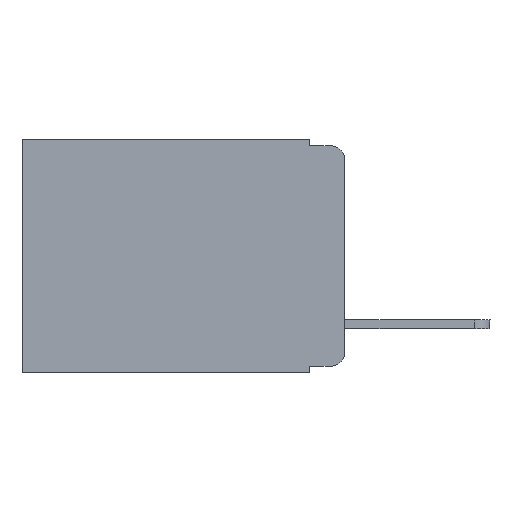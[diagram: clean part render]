
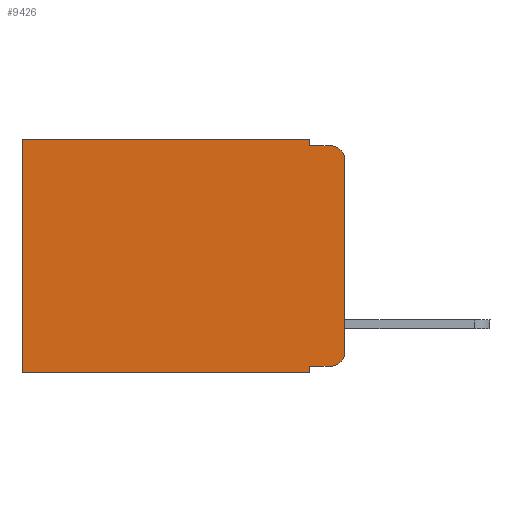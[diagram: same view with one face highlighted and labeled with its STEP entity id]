
A CAD part, left-side view. The second image highlights one B-rep face of the part: STEP entity #9426.
In plain terms, the highlighted planar face has unit normal (-1, 0, 0).
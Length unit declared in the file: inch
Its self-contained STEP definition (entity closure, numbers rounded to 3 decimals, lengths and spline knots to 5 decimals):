
#676 = LINE ( 'NONE', #734, #9993 ) ;
#734 = CARTESIAN_POINT ( 'NONE',  ( 0.298, 0.051, 0. ) ) ;
#769 = LINE ( 'NONE', #6448, #11673 ) ;
#831 = VERTEX_POINT ( 'NONE', #12209 ) ;
#836 = VERTEX_POINT ( 'NONE', #8332 ) ;
#1305 = AXIS2_PLACEMENT_3D ( 'NONE', #5976, #6216, #8032 ) ;
#1352 = CARTESIAN_POINT ( 'NONE',  ( 0.298, 0.473, -0.343 ) ) ;
#1422 = CARTESIAN_POINT ( 'NONE',  ( 0.298, 0.02, -0.01 ) ) ;
#1475 = VERTEX_POINT ( 'NONE', #4830 ) ;
#1585 = EDGE_CURVE ( 'NONE', #836, #831, #676, .T. ) ;
#1597 = DIRECTION ( 'NONE',  ( -1., 0., 0. ) ) ;
#1700 = EDGE_CURVE ( 'NONE', #8218, #3048, #10352, .T. ) ;
#1705 = VERTEX_POINT ( 'NONE', #7664 ) ;
#1864 = CARTESIAN_POINT ( 'NONE',  ( 0.298, 0., -0.313 ) ) ;
#1930 = DIRECTION ( 'NONE',  ( 0., 0., -1. ) ) ;
#2500 = DIRECTION ( 'NONE',  ( 0., 0., -1. ) ) ;
#2582 = DIRECTION ( 'NONE',  ( 0., 0., -1. ) ) ;
#2620 = AXIS2_PLACEMENT_3D ( 'NONE', #11358, #2967, #1930 ) ;
#2673 = CARTESIAN_POINT ( 'NONE',  ( 0.298, 0.051, -0.333 ) ) ;
#2722 = ORIENTED_EDGE ( 'NONE', *, *, #8827, .F. ) ;
#2781 = VECTOR ( 'NONE', #6067, 39.37008 ) ;
#2967 = DIRECTION ( 'NONE',  ( 1., 0., 0. ) ) ;
#3048 = VERTEX_POINT ( 'NONE', #1864 ) ;
#3181 = LINE ( 'NONE', #7083, #3971 ) ;
#3281 = VECTOR ( 'NONE', #6327, 39.37008 ) ;
#3443 = VERTEX_POINT ( 'NONE', #1422 ) ;
#3461 = VERTEX_POINT ( 'NONE', #10984 ) ;
#3486 = CARTESIAN_POINT ( 'NONE',  ( 0.298, 0.051, -0.01 ) ) ;
#3590 = PLANE ( 'NONE',  #2620 ) ;
#3823 = EDGE_CURVE ( 'NONE', #1705, #3443, #9048, .T. ) ;
#3971 = VECTOR ( 'NONE', #8991, 39.37008 ) ;
#4249 = CIRCLE ( 'NONE', #1305, 0.02 ) ;
#4801 = EDGE_CURVE ( 'NONE', #8218, #3443, #4249, .T. ) ;
#4830 = CARTESIAN_POINT ( 'NONE',  ( 0.298, 0.02, -0.333 ) ) ;
#5017 = LINE ( 'NONE', #11632, #2781 ) ;
#5194 = VECTOR ( 'NONE', #12122, 39.37008 ) ;
#5557 = LINE ( 'NONE', #11180, #10906 ) ;
#5901 = ORIENTED_EDGE ( 'NONE', *, *, #8743, .F. ) ;
#5976 = CARTESIAN_POINT ( 'NONE',  ( 0.298, 0.02, -0.03 ) ) ;
#6017 = CARTESIAN_POINT ( 'NONE',  ( 0.298, 0.051, 0. ) ) ;
#6067 = DIRECTION ( 'NONE',  ( 0., 1., 0. ) ) ;
#6143 = CIRCLE ( 'NONE', #8146, 0.02 ) ;
#6216 = DIRECTION ( 'NONE',  ( -1., 0., 0. ) ) ;
#6327 = DIRECTION ( 'NONE',  ( 0., -1., 0. ) ) ;
#6448 = CARTESIAN_POINT ( 'NONE',  ( 0.298, 0.051, 0. ) ) ;
#6751 = ORIENTED_EDGE ( 'NONE', *, *, #7006, .T. ) ;
#7006 = EDGE_CURVE ( 'NONE', #10038, #3461, #5017, .T. ) ;
#7079 = CARTESIAN_POINT ( 'NONE',  ( 0.298, 0., -0.03 ) ) ;
#7083 = CARTESIAN_POINT ( 'NONE',  ( 0.298, 0., -0.343 ) ) ;
#7356 = ORIENTED_EDGE ( 'NONE', *, *, #4801, .T. ) ;
#7437 = DIRECTION ( 'NONE',  ( 0., 0., -1. ) ) ;
#7639 = ORIENTED_EDGE ( 'NONE', *, *, #10543, .T. ) ;
#7664 = CARTESIAN_POINT ( 'NONE',  ( 0.298, 0.051, -0.01 ) ) ;
#7813 = VECTOR ( 'NONE', #9424, 39.37008 ) ;
#8032 = DIRECTION ( 'NONE',  ( 0., 0., -1. ) ) ;
#8146 = AXIS2_PLACEMENT_3D ( 'NONE', #12151, #1597, #2582 ) ;
#8185 = LINE ( 'NONE', #2673, #5194 ) ;
#8218 = VERTEX_POINT ( 'NONE', #7079 ) ;
#8332 = CARTESIAN_POINT ( 'NONE',  ( 0.298, 0.051, -0.333 ) ) ;
#8424 = EDGE_CURVE ( 'NONE', #1475, #3048, #6143, .T. ) ;
#8588 = CARTESIAN_POINT ( 'NONE',  ( 0.298, 0., 0. ) ) ;
#8743 = EDGE_CURVE ( 'NONE', #831, #11243, #3181, .T. ) ;
#8827 = EDGE_CURVE ( 'NONE', #10038, #1705, #769, .T. ) ;
#8991 = DIRECTION ( 'NONE',  ( 0., 1., 0. ) ) ;
#9048 = LINE ( 'NONE', #3486, #3281 ) ;
#9159 = ORIENTED_EDGE ( 'NONE', *, *, #1700, .F. ) ;
#9424 = DIRECTION ( 'NONE',  ( 0., 0., -1. ) ) ;
#9426 = ADVANCED_FACE ( 'NONE', ( #11062 ), #3590, .F. ) ;
#9630 = ORIENTED_EDGE ( 'NONE', *, *, #1585, .F. ) ;
#9695 = DIRECTION ( 'NONE',  ( 0., 0., -1. ) ) ;
#9993 = VECTOR ( 'NONE', #9695, 39.37008 ) ;
#10038 = VERTEX_POINT ( 'NONE', #6017 ) ;
#10352 = LINE ( 'NONE', #8588, #7813 ) ;
#10543 = EDGE_CURVE ( 'NONE', #836, #1475, #8185, .T. ) ;
#10585 = ORIENTED_EDGE ( 'NONE', *, *, #3823, .F. ) ;
#10622 = EDGE_CURVE ( 'NONE', #3461, #11243, #5557, .T. ) ;
#10878 = ORIENTED_EDGE ( 'NONE', *, *, #10622, .T. ) ;
#10906 = VECTOR ( 'NONE', #7437, 39.37008 ) ;
#10958 = ORIENTED_EDGE ( 'NONE', *, *, #8424, .T. ) ;
#10984 = CARTESIAN_POINT ( 'NONE',  ( 0.298, 0.473, 0. ) ) ;
#11062 = FACE_OUTER_BOUND ( 'NONE', #12202, .T. ) ;
#11180 = CARTESIAN_POINT ( 'NONE',  ( 0.298, 0.473, 0. ) ) ;
#11243 = VERTEX_POINT ( 'NONE', #1352 ) ;
#11358 = CARTESIAN_POINT ( 'NONE',  ( 0.298, 0., 0. ) ) ;
#11632 = CARTESIAN_POINT ( 'NONE',  ( 0.298, 0., 0. ) ) ;
#11673 = VECTOR ( 'NONE', #2500, 39.37008 ) ;
#12122 = DIRECTION ( 'NONE',  ( 0., -1., 0. ) ) ;
#12151 = CARTESIAN_POINT ( 'NONE',  ( 0.298, 0.02, -0.313 ) ) ;
#12202 = EDGE_LOOP ( 'NONE', ( #9159, #7356, #10585, #2722, #6751, #10878, #5901, #9630, #7639, #10958 ) ) ;
#12209 = CARTESIAN_POINT ( 'NONE',  ( 0.298, 0.051, -0.343 ) ) ;
